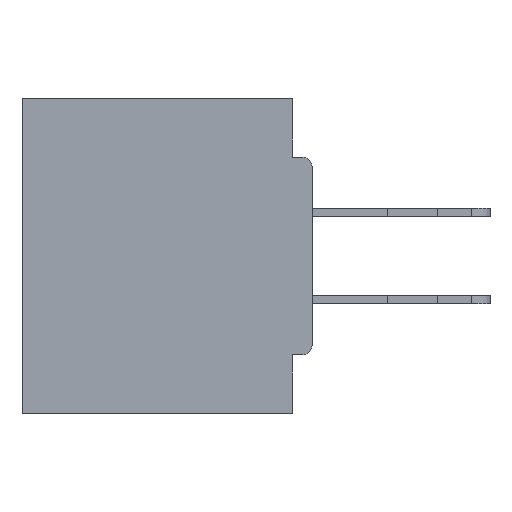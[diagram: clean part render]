
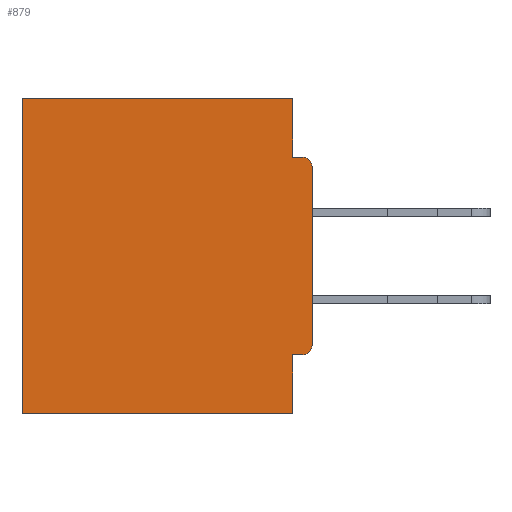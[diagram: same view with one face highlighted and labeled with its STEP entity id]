
A CAD part, left-side view. The second image highlights one B-rep face of the part: STEP entity #879.
In plain terms, the highlighted planar face has unit normal (-1, 0, 0).
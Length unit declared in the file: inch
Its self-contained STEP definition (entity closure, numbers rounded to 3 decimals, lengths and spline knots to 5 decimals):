
#109 = AXIS2_PLACEMENT_3D ( 'NONE', #2503, #2753, #8171 ) ;
#651 = LINE ( 'NONE', #7988, #29738 ) ;
#879 = ADVANCED_FACE ( 'NONE', ( #18991 ), #15826, .F. ) ;
#1174 = CIRCLE ( 'NONE', #17970, 0.015 ) ;
#1649 = LINE ( 'NONE', #25084, #6974 ) ;
#1934 = EDGE_CURVE ( 'NONE', #35795, #18028, #29132, .T. ) ;
#2503 = CARTESIAN_POINT ( 'NONE',  ( 0.298, 0.015, -0.1085 ) ) ;
#2753 = DIRECTION ( 'NONE',  ( -1., 0., 0. ) ) ;
#2816 = AXIS2_PLACEMENT_3D ( 'NONE', #35655, #24499, #18663 ) ;
#3255 = EDGE_CURVE ( 'NONE', #17441, #22034, #1649, .T. ) ;
#4833 = DIRECTION ( 'NONE',  ( 0., 0., -1. ) ) ;
#5056 = ORIENTED_EDGE ( 'NONE', *, *, #23048, .F. ) ;
#5425 = CARTESIAN_POINT ( 'NONE',  ( 0.298, 0., -0.0935 ) ) ;
#5522 = DIRECTION ( 'NONE',  ( 0., 0., -1. ) ) ;
#5635 = ORIENTED_EDGE ( 'NONE', *, *, #1934, .T. ) ;
#6026 = ORIENTED_EDGE ( 'NONE', *, *, #3255, .F. ) ;
#6147 = EDGE_CURVE ( 'NONE', #31225, #21385, #35716, .T. ) ;
#6222 = LINE ( 'NONE', #7060, #36262 ) ;
#6951 = DIRECTION ( 'NONE',  ( 0., 1., 0. ) ) ;
#6974 = VECTOR ( 'NONE', #5522, 39.37008 ) ;
#7060 = CARTESIAN_POINT ( 'NONE',  ( 0.298, 0., -0.5 ) ) ;
#7438 = EDGE_CURVE ( 'NONE', #23438, #21385, #1174, .T. ) ;
#7988 = CARTESIAN_POINT ( 'NONE',  ( 0.298, 0.031, -0.5 ) ) ;
#8076 = CARTESIAN_POINT ( 'NONE',  ( 0.298, 0.46, -0.5 ) ) ;
#8171 = DIRECTION ( 'NONE',  ( 0., 0., -1. ) ) ;
#8234 = CARTESIAN_POINT ( 'NONE',  ( 0.298, 0.46, 0. ) ) ;
#9069 = EDGE_CURVE ( 'NONE', #23438, #17441, #31516, .T. ) ;
#10182 = ORIENTED_EDGE ( 'NONE', *, *, #7438, .T. ) ;
#10422 = DIRECTION ( 'NONE',  ( -1., 0., 0. ) ) ;
#10805 = ORIENTED_EDGE ( 'NONE', *, *, #30327, .F. ) ;
#10990 = ORIENTED_EDGE ( 'NONE', *, *, #9069, .F. ) ;
#11180 = CARTESIAN_POINT ( 'NONE',  ( 0.298, 0., -0.3915 ) ) ;
#11208 = DIRECTION ( 'NONE',  ( 0., -1., 0. ) ) ;
#11412 = VECTOR ( 'NONE', #4833, 39.37008 ) ;
#12559 = VECTOR ( 'NONE', #13624, 39.37008 ) ;
#12618 = CARTESIAN_POINT ( 'NONE',  ( 0.298, 0., -0.1085 ) ) ;
#13624 = DIRECTION ( 'NONE',  ( 0., 0., -1. ) ) ;
#14013 = DIRECTION ( 'NONE',  ( 0., 1., 0. ) ) ;
#15826 = PLANE ( 'NONE',  #2816 ) ;
#15837 = CARTESIAN_POINT ( 'NONE',  ( 0.298, 0.031, -0.5 ) ) ;
#15843 = ORIENTED_EDGE ( 'NONE', *, *, #6147, .F. ) ;
#16219 = DIRECTION ( 'NONE',  ( 0., 1., 0. ) ) ;
#16578 = CARTESIAN_POINT ( 'NONE',  ( 0.298, 0.031, 0. ) ) ;
#17441 = VERTEX_POINT ( 'NONE', #29211 ) ;
#17876 = VERTEX_POINT ( 'NONE', #20787 ) ;
#17890 = CIRCLE ( 'NONE', #109, 0.015 ) ;
#17970 = AXIS2_PLACEMENT_3D ( 'NONE', #19181, #10422, #33382 ) ;
#18028 = VERTEX_POINT ( 'NONE', #23995 ) ;
#18663 = DIRECTION ( 'NONE',  ( 0., 0., -1. ) ) ;
#18721 = VECTOR ( 'NONE', #11208, 39.37008 ) ;
#18991 = FACE_OUTER_BOUND ( 'NONE', #19409, .T. ) ;
#19181 = CARTESIAN_POINT ( 'NONE',  ( 0.298, 0.015, -0.3915 ) ) ;
#19260 = EDGE_CURVE ( 'NONE', #22034, #27364, #6222, .T. ) ;
#19409 = EDGE_LOOP ( 'NONE', ( #34604, #10805, #5056, #5635, #20152, #31774, #6026, #10990, #10182, #15843 ) ) ;
#20152 = ORIENTED_EDGE ( 'NONE', *, *, #23085, .T. ) ;
#20681 = VECTOR ( 'NONE', #16219, 39.37008 ) ;
#20787 = CARTESIAN_POINT ( 'NONE',  ( 0.298, 0.031, -0.0935 ) ) ;
#21385 = VERTEX_POINT ( 'NONE', #11180 ) ;
#22034 = VERTEX_POINT ( 'NONE', #15837 ) ;
#22351 = CARTESIAN_POINT ( 'NONE',  ( 0.298, 0.015, -0.4065 ) ) ;
#22647 = CARTESIAN_POINT ( 'NONE',  ( 0.298, 0., -0.4065 ) ) ;
#23048 = EDGE_CURVE ( 'NONE', #35795, #17876, #651, .T. ) ;
#23085 = EDGE_CURVE ( 'NONE', #18028, #27364, #32419, .T. ) ;
#23438 = VERTEX_POINT ( 'NONE', #22351 ) ;
#23995 = CARTESIAN_POINT ( 'NONE',  ( 0.298, 0.46, 0. ) ) ;
#24499 = DIRECTION ( 'NONE',  ( 1., 0., 0. ) ) ;
#24739 = DIRECTION ( 'NONE',  ( 0., 0., -1. ) ) ;
#24773 = CARTESIAN_POINT ( 'NONE',  ( 0.298, 0., 0. ) ) ;
#24914 = LINE ( 'NONE', #5425, #18721 ) ;
#25084 = CARTESIAN_POINT ( 'NONE',  ( 0.298, 0.031, -0.5 ) ) ;
#25468 = VERTEX_POINT ( 'NONE', #25870 ) ;
#25870 = CARTESIAN_POINT ( 'NONE',  ( 0.298, 0.015, -0.0935 ) ) ;
#27364 = VERTEX_POINT ( 'NONE', #8076 ) ;
#29132 = LINE ( 'NONE', #32808, #20681 ) ;
#29211 = CARTESIAN_POINT ( 'NONE',  ( 0.298, 0.031, -0.4065 ) ) ;
#29738 = VECTOR ( 'NONE', #24739, 39.37008 ) ;
#30327 = EDGE_CURVE ( 'NONE', #17876, #25468, #24914, .T. ) ;
#31225 = VERTEX_POINT ( 'NONE', #12618 ) ;
#31516 = LINE ( 'NONE', #22647, #35975 ) ;
#31774 = ORIENTED_EDGE ( 'NONE', *, *, #19260, .F. ) ;
#32419 = LINE ( 'NONE', #8234, #12559 ) ;
#32808 = CARTESIAN_POINT ( 'NONE',  ( 0.298, 0., 0. ) ) ;
#33382 = DIRECTION ( 'NONE',  ( 0., 0., -1. ) ) ;
#34604 = ORIENTED_EDGE ( 'NONE', *, *, #36349, .T. ) ;
#35655 = CARTESIAN_POINT ( 'NONE',  ( 0.298, 0., 0. ) ) ;
#35716 = LINE ( 'NONE', #24773, #11412 ) ;
#35795 = VERTEX_POINT ( 'NONE', #16578 ) ;
#35975 = VECTOR ( 'NONE', #14013, 39.37008 ) ;
#36262 = VECTOR ( 'NONE', #6951, 39.37008 ) ;
#36349 = EDGE_CURVE ( 'NONE', #31225, #25468, #17890, .T. ) ;
